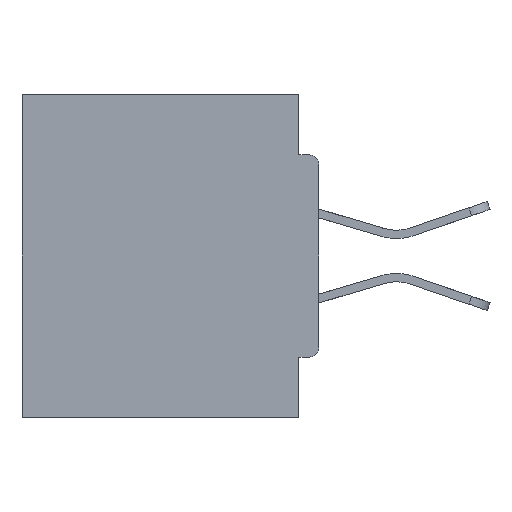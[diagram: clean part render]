
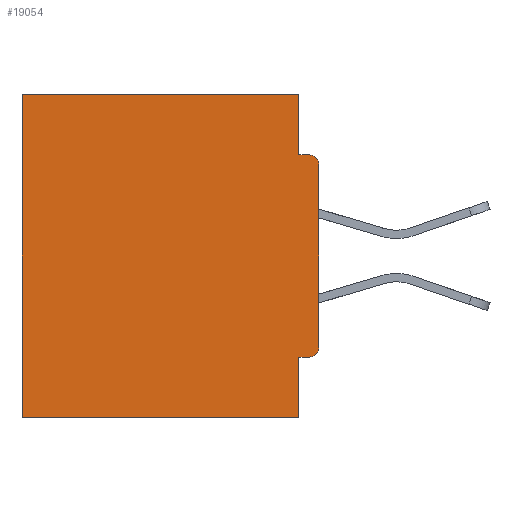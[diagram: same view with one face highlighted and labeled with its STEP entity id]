
A CAD part, left-side view. The second image highlights one B-rep face of the part: STEP entity #19054.
In plain terms, the highlighted planar face has unit normal (-1, 0, 0).
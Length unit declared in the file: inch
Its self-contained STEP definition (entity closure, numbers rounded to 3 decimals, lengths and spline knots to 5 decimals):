
#47 = EDGE_CURVE ( 'NONE', #21165, #33172, #16275, .T. ) ;
#178 = VERTEX_POINT ( 'NONE', #12140 ) ;
#303 = DIRECTION ( 'NONE',  ( 0., 0., -1. ) ) ;
#551 = CARTESIAN_POINT ( 'NONE',  ( 0.298, 0.031, -0.4065 ) ) ;
#707 = DIRECTION ( 'NONE',  ( 0., 0., -1. ) ) ;
#847 = CIRCLE ( 'NONE', #35091, 0.015 ) ;
#979 = DIRECTION ( 'NONE',  ( 0., 1., 0. ) ) ;
#1225 = CARTESIAN_POINT ( 'NONE',  ( 0.298, 0.46, -0.5 ) ) ;
#3371 = LINE ( 'NONE', #26499, #14675 ) ;
#3789 = DIRECTION ( 'NONE',  ( 1., 0., 0. ) ) ;
#3819 = ORIENTED_EDGE ( 'NONE', *, *, #20883, .F. ) ;
#4439 = ORIENTED_EDGE ( 'NONE', *, *, #16198, .F. ) ;
#4500 = VECTOR ( 'NONE', #6679, 39.37008 ) ;
#4775 = CARTESIAN_POINT ( 'NONE',  ( 0.298, 0.015, -0.0935 ) ) ;
#5470 = VECTOR ( 'NONE', #19479, 39.37008 ) ;
#5679 = ORIENTED_EDGE ( 'NONE', *, *, #13869, .F. ) ;
#6044 = LINE ( 'NONE', #33566, #28303 ) ;
#6097 = CARTESIAN_POINT ( 'NONE',  ( 0.298, 0.46, 0. ) ) ;
#6228 = CARTESIAN_POINT ( 'NONE',  ( 0.298, 0.015, -0.3915 ) ) ;
#6394 = EDGE_CURVE ( 'NONE', #178, #32007, #8444, .T. ) ;
#6679 = DIRECTION ( 'NONE',  ( 0., -1., 0. ) ) ;
#7607 = CARTESIAN_POINT ( 'NONE',  ( 0.298, 0.031, -0.5 ) ) ;
#7733 = CARTESIAN_POINT ( 'NONE',  ( 0.298, 0.031, -0.0935 ) ) ;
#8436 = DIRECTION ( 'NONE',  ( 0., 0., -1. ) ) ;
#8444 = LINE ( 'NONE', #18210, #25901 ) ;
#9391 = CARTESIAN_POINT ( 'NONE',  ( 0.298, 0., -0.3915 ) ) ;
#9697 = FACE_OUTER_BOUND ( 'NONE', #24872, .T. ) ;
#11018 = ORIENTED_EDGE ( 'NONE', *, *, #23609, .F. ) ;
#11428 = CARTESIAN_POINT ( 'NONE',  ( 0.298, 0.015, -0.1085 ) ) ;
#12140 = CARTESIAN_POINT ( 'NONE',  ( 0.298, 0.015, -0.4065 ) ) ;
#12677 = EDGE_CURVE ( 'NONE', #35721, #33172, #20181, .T. ) ;
#13034 = AXIS2_PLACEMENT_3D ( 'NONE', #23014, #3789, #34157 ) ;
#13869 = EDGE_CURVE ( 'NONE', #31877, #35721, #25764, .T. ) ;
#14091 = DIRECTION ( 'NONE',  ( -1., 0., 0. ) ) ;
#14625 = CARTESIAN_POINT ( 'NONE',  ( 0.298, 0.46, 0. ) ) ;
#14675 = VECTOR ( 'NONE', #979, 39.37008 ) ;
#15235 = VERTEX_POINT ( 'NONE', #7607 ) ;
#15463 = EDGE_CURVE ( 'NONE', #31347, #22657, #20850, .T. ) ;
#16198 = EDGE_CURVE ( 'NONE', #21165, #20035, #18630, .T. ) ;
#16275 = CIRCLE ( 'NONE', #16323, 0.015 ) ;
#16323 = AXIS2_PLACEMENT_3D ( 'NONE', #11428, #14091, #303 ) ;
#17662 = LINE ( 'NONE', #33302, #5470 ) ;
#18210 = CARTESIAN_POINT ( 'NONE',  ( 0.298, 0., -0.4065 ) ) ;
#18630 = LINE ( 'NONE', #35346, #19483 ) ;
#18857 = ORIENTED_EDGE ( 'NONE', *, *, #15463, .T. ) ;
#18969 = ORIENTED_EDGE ( 'NONE', *, *, #33100, .T. ) ;
#19054 = ADVANCED_FACE ( 'NONE', ( #9697 ), #34655, .F. ) ;
#19114 = VECTOR ( 'NONE', #707, 39.37008 ) ;
#19479 = DIRECTION ( 'NONE',  ( 0., 1., 0. ) ) ;
#19483 = VECTOR ( 'NONE', #24063, 39.37008 ) ;
#19924 = CARTESIAN_POINT ( 'NONE',  ( 0.298, 0.031, -0.5 ) ) ;
#20035 = VERTEX_POINT ( 'NONE', #9391 ) ;
#20181 = LINE ( 'NONE', #28366, #4500 ) ;
#20850 = LINE ( 'NONE', #14625, #19114 ) ;
#20883 = EDGE_CURVE ( 'NONE', #32007, #15235, #6044, .T. ) ;
#21165 = VERTEX_POINT ( 'NONE', #25429 ) ;
#22657 = VERTEX_POINT ( 'NONE', #1225 ) ;
#23014 = CARTESIAN_POINT ( 'NONE',  ( 0.298, 0., 0. ) ) ;
#23581 = DIRECTION ( 'NONE',  ( 0., 0., -1. ) ) ;
#23609 = EDGE_CURVE ( 'NONE', #15235, #22657, #17662, .T. ) ;
#24063 = DIRECTION ( 'NONE',  ( 0., 0., -1. ) ) ;
#24872 = EDGE_LOOP ( 'NONE', ( #29819, #28799, #5679, #18969, #18857, #11018, #3819, #29967, #32435, #4439 ) ) ;
#25429 = CARTESIAN_POINT ( 'NONE',  ( 0.298, 0., -0.1085 ) ) ;
#25764 = LINE ( 'NONE', #19924, #29687 ) ;
#25901 = VECTOR ( 'NONE', #29791, 39.37008 ) ;
#26499 = CARTESIAN_POINT ( 'NONE',  ( 0.298, 0., 0. ) ) ;
#28303 = VECTOR ( 'NONE', #32840, 39.37008 ) ;
#28366 = CARTESIAN_POINT ( 'NONE',  ( 0.298, 0., -0.0935 ) ) ;
#28799 = ORIENTED_EDGE ( 'NONE', *, *, #12677, .F. ) ;
#29687 = VECTOR ( 'NONE', #23581, 39.37008 ) ;
#29791 = DIRECTION ( 'NONE',  ( 0., 1., 0. ) ) ;
#29819 = ORIENTED_EDGE ( 'NONE', *, *, #47, .T. ) ;
#29967 = ORIENTED_EDGE ( 'NONE', *, *, #6394, .F. ) ;
#31347 = VERTEX_POINT ( 'NONE', #6097 ) ;
#31426 = EDGE_CURVE ( 'NONE', #178, #20035, #847, .T. ) ;
#31877 = VERTEX_POINT ( 'NONE', #34110 ) ;
#32007 = VERTEX_POINT ( 'NONE', #551 ) ;
#32435 = ORIENTED_EDGE ( 'NONE', *, *, #31426, .T. ) ;
#32840 = DIRECTION ( 'NONE',  ( 0., 0., -1. ) ) ;
#33100 = EDGE_CURVE ( 'NONE', #31877, #31347, #3371, .T. ) ;
#33172 = VERTEX_POINT ( 'NONE', #4775 ) ;
#33302 = CARTESIAN_POINT ( 'NONE',  ( 0.298, 0., -0.5 ) ) ;
#33566 = CARTESIAN_POINT ( 'NONE',  ( 0.298, 0.031, -0.5 ) ) ;
#33668 = DIRECTION ( 'NONE',  ( -1., 0., 0. ) ) ;
#34110 = CARTESIAN_POINT ( 'NONE',  ( 0.298, 0.031, 0. ) ) ;
#34157 = DIRECTION ( 'NONE',  ( 0., 0., -1. ) ) ;
#34655 = PLANE ( 'NONE',  #13034 ) ;
#35091 = AXIS2_PLACEMENT_3D ( 'NONE', #6228, #33668, #8436 ) ;
#35346 = CARTESIAN_POINT ( 'NONE',  ( 0.298, 0., 0. ) ) ;
#35721 = VERTEX_POINT ( 'NONE', #7733 ) ;
